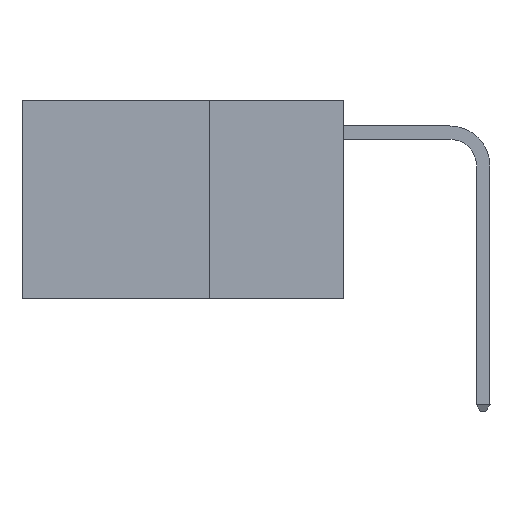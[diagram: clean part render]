
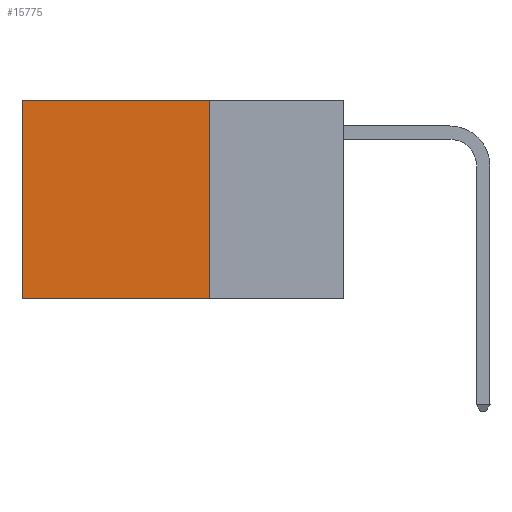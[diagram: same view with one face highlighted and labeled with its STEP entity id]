
A CAD part, left-side view. The second image highlights one B-rep face of the part: STEP entity #15775.
In plain terms, the highlighted planar face has unit normal (-1, 0, 0).
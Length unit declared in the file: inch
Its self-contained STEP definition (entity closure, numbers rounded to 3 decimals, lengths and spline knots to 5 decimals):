
#438 = CARTESIAN_POINT ( 'NONE',  ( 0.2625, 0.25, 0. ) ) ;
#1405 = ORIENTED_EDGE ( 'NONE', *, *, #11363, .T. ) ;
#1918 = CARTESIAN_POINT ( 'NONE',  ( 0.2625, 0.25, -0.37 ) ) ;
#2149 = EDGE_LOOP ( 'NONE', ( #1405, #26258, #24865, #24225 ) ) ;
#2395 = VECTOR ( 'NONE', #17217, 39.37008 ) ;
#2587 = EDGE_CURVE ( 'NONE', #13714, #23511, #19153, .T. ) ;
#2608 = DIRECTION ( 'NONE',  ( 0., 0., -1. ) ) ;
#2814 = CARTESIAN_POINT ( 'NONE',  ( 0.2625, 0.25, 0. ) ) ;
#2828 = DIRECTION ( 'NONE',  ( 0., 0., -1. ) ) ;
#3361 = FACE_OUTER_BOUND ( 'NONE', #2149, .T. ) ;
#4667 = VERTEX_POINT ( 'NONE', #6836 ) ;
#6836 = CARTESIAN_POINT ( 'NONE',  ( 0.2625, 0.6, 0. ) ) ;
#8560 = LINE ( 'NONE', #10301, #2395 ) ;
#10301 = CARTESIAN_POINT ( 'NONE',  ( 0.2625, 0.25, 0. ) ) ;
#11363 = EDGE_CURVE ( 'NONE', #4667, #28732, #15495, .T. ) ;
#12032 = PLANE ( 'NONE',  #23355 ) ;
#12583 = VECTOR ( 'NONE', #12731, 39.37008 ) ;
#12731 = DIRECTION ( 'NONE',  ( 0., 1., 0. ) ) ;
#13714 = VERTEX_POINT ( 'NONE', #18523 ) ;
#15495 = LINE ( 'NONE', #18575, #26745 ) ;
#15775 = ADVANCED_FACE ( 'NONE', ( #3361 ), #12032, .F. ) ;
#16620 = DIRECTION ( 'NONE',  ( 1., 0., 0. ) ) ;
#17217 = DIRECTION ( 'NONE',  ( 0., 1., 0. ) ) ;
#18445 = VECTOR ( 'NONE', #2608, 39.37008 ) ;
#18523 = CARTESIAN_POINT ( 'NONE',  ( 0.2625, 0.25, 0. ) ) ;
#18575 = CARTESIAN_POINT ( 'NONE',  ( 0.2625, 0.6, 0. ) ) ;
#19153 = LINE ( 'NONE', #2814, #18445 ) ;
#19327 = LINE ( 'NONE', #24080, #12583 ) ;
#20889 = DIRECTION ( 'NONE',  ( 0., 0., -1. ) ) ;
#21941 = EDGE_CURVE ( 'NONE', #13714, #4667, #8560, .T. ) ;
#23117 = CARTESIAN_POINT ( 'NONE',  ( 0.2625, 0.6, -0.37 ) ) ;
#23355 = AXIS2_PLACEMENT_3D ( 'NONE', #438, #16620, #2828 ) ;
#23511 = VERTEX_POINT ( 'NONE', #1918 ) ;
#24080 = CARTESIAN_POINT ( 'NONE',  ( 0.2625, 0.25, -0.37 ) ) ;
#24225 = ORIENTED_EDGE ( 'NONE', *, *, #21941, .T. ) ;
#24865 = ORIENTED_EDGE ( 'NONE', *, *, #2587, .F. ) ;
#26258 = ORIENTED_EDGE ( 'NONE', *, *, #27162, .F. ) ;
#26745 = VECTOR ( 'NONE', #20889, 39.37008 ) ;
#27162 = EDGE_CURVE ( 'NONE', #23511, #28732, #19327, .T. ) ;
#28732 = VERTEX_POINT ( 'NONE', #23117 ) ;
